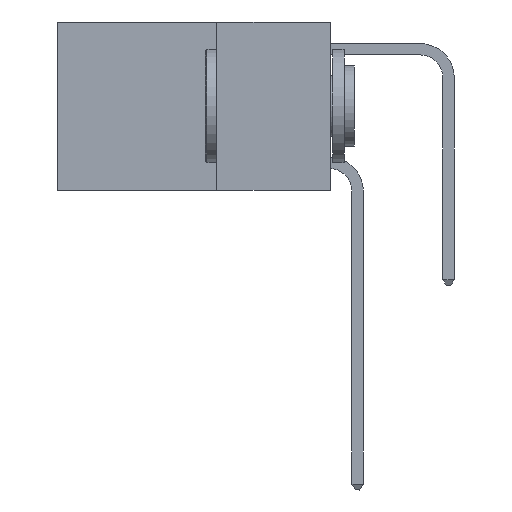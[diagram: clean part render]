
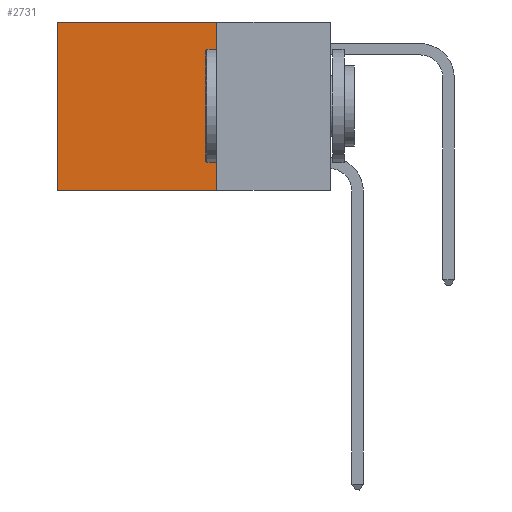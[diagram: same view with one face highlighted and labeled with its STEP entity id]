
A CAD part, left-side view. The second image highlights one B-rep face of the part: STEP entity #2731.
In plain terms, the highlighted planar face has unit normal (-1, 0, 0).
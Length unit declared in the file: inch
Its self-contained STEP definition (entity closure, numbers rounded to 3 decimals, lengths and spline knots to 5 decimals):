
#754 = CARTESIAN_POINT ( 'NONE',  ( 0.2625, 0.6, 0. ) ) ;
#2101 = VECTOR ( 'NONE', #28877, 39.37008 ) ;
#2666 = DIRECTION ( 'NONE',  ( 0., 0., -1. ) ) ;
#2731 = ADVANCED_FACE ( 'NONE', ( #4921 ), #2962, .F. ) ;
#2962 = PLANE ( 'NONE',  #20504 ) ;
#3850 = DIRECTION ( 'NONE',  ( 0., 1., 0. ) ) ;
#4701 = CARTESIAN_POINT ( 'NONE',  ( 0.2625, 0.6, -0.37 ) ) ;
#4921 = FACE_OUTER_BOUND ( 'NONE', #11161, .T. ) ;
#5247 = EDGE_CURVE ( 'NONE', #7231, #7852, #24016, .T. ) ;
#7231 = VERTEX_POINT ( 'NONE', #13180 ) ;
#7310 = VERTEX_POINT ( 'NONE', #4701 ) ;
#7687 = CARTESIAN_POINT ( 'NONE',  ( 0.2625, 0.25, -0.37 ) ) ;
#7852 = VERTEX_POINT ( 'NONE', #7687 ) ;
#10060 = CARTESIAN_POINT ( 'NONE',  ( 0.2625, 0.25, 0. ) ) ;
#10477 = CARTESIAN_POINT ( 'NONE',  ( 0.2625, 0.25, -0.37 ) ) ;
#11161 = EDGE_LOOP ( 'NONE', ( #13631, #14824, #19637, #20259 ) ) ;
#12222 = EDGE_CURVE ( 'NONE', #7231, #12793, #29622, .T. ) ;
#12546 = CARTESIAN_POINT ( 'NONE',  ( 0.2625, 0.25, 0. ) ) ;
#12793 = VERTEX_POINT ( 'NONE', #16008 ) ;
#13180 = CARTESIAN_POINT ( 'NONE',  ( 0.2625, 0.25, 0. ) ) ;
#13631 = ORIENTED_EDGE ( 'NONE', *, *, #24624, .T. ) ;
#14133 = DIRECTION ( 'NONE',  ( 1., 0., 0. ) ) ;
#14824 = ORIENTED_EDGE ( 'NONE', *, *, #19941, .F. ) ;
#16008 = CARTESIAN_POINT ( 'NONE',  ( 0.2625, 0.6, 0. ) ) ;
#16818 = VECTOR ( 'NONE', #3850, 39.37008 ) ;
#19146 = DIRECTION ( 'NONE',  ( 0., 0., -1. ) ) ;
#19637 = ORIENTED_EDGE ( 'NONE', *, *, #5247, .F. ) ;
#19766 = DIRECTION ( 'NONE',  ( 0., 0., -1. ) ) ;
#19941 = EDGE_CURVE ( 'NONE', #7852, #7310, #24043, .T. ) ;
#20259 = ORIENTED_EDGE ( 'NONE', *, *, #12222, .T. ) ;
#20504 = AXIS2_PLACEMENT_3D ( 'NONE', #10060, #14133, #2666 ) ;
#22542 = CARTESIAN_POINT ( 'NONE',  ( 0.2625, 0.25, 0. ) ) ;
#24016 = LINE ( 'NONE', #12546, #26505 ) ;
#24043 = LINE ( 'NONE', #10477, #2101 ) ;
#24624 = EDGE_CURVE ( 'NONE', #12793, #7310, #28527, .T. ) ;
#26505 = VECTOR ( 'NONE', #19766, 39.37008 ) ;
#28527 = LINE ( 'NONE', #754, #29471 ) ;
#28877 = DIRECTION ( 'NONE',  ( 0., 1., 0. ) ) ;
#29471 = VECTOR ( 'NONE', #19146, 39.37008 ) ;
#29622 = LINE ( 'NONE', #22542, #16818 ) ;
